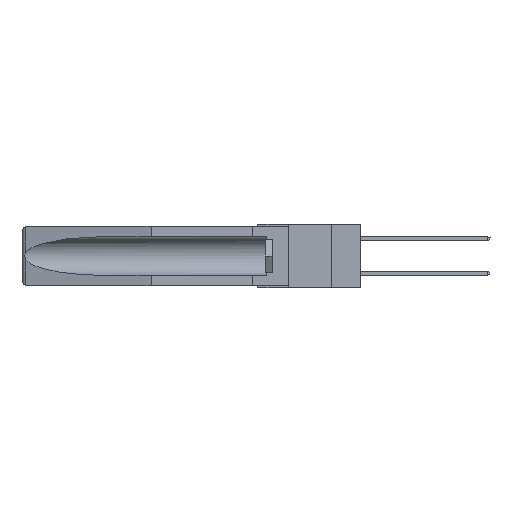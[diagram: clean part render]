
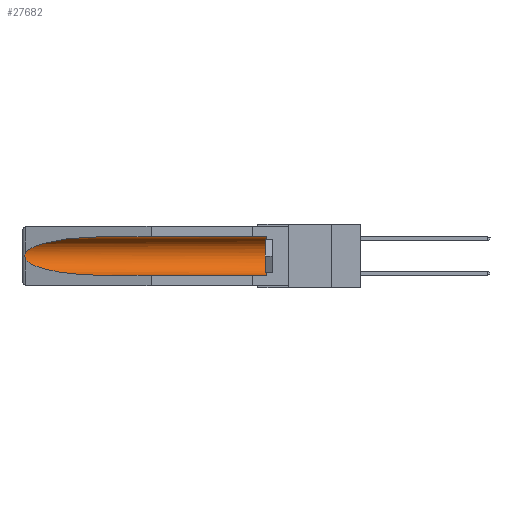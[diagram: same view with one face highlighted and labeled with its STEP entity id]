
A CAD part, left-side view. The second image highlights one B-rep face of the part: STEP entity #27682.
In plain terms, the highlighted cylindrical face has radius 2.857 mm (diameter 5.715 mm), a partial arc.
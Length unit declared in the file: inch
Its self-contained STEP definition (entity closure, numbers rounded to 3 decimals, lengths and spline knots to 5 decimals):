
#63 = DIRECTION ( 'NONE',  ( 0., 1., 0. ) ) ;
#552 = CARTESIAN_POINT ( 'NONE',  ( 0.26537, 1.52718, -0.14972 ) ) ;
#564 = VERTEX_POINT ( 'NONE', #11692 ) ;
#1030 = CARTESIAN_POINT ( 'NONE',  ( 0.155, 0.126, -0.1715 ) ) ;
#1055 = ORIENTED_EDGE ( 'NONE', *, *, #6810, .T. ) ;
#1767 = VECTOR ( 'NONE', #63, 39.37008 ) ;
#1790 = ORIENTED_EDGE ( 'NONE', *, *, #19534, .T. ) ;
#1991 = LINE ( 'NONE', #5428, #10099 ) ;
#2625 = EDGE_LOOP ( 'NONE', ( #1055, #1790, #20325, #8831, #15726, #8059 ) ) ;
#3124 = CARTESIAN_POINT ( 'NONE',  ( 0.26597, 1.5296, -0.19026 ) ) ;
#3127 = FACE_OUTER_BOUND ( 'NONE', #2625, .T. ) ;
#4178 = CARTESIAN_POINT ( 'NONE',  ( 0.155, 0.126, -0.059 ) ) ;
#4652 = CARTESIAN_POINT ( 'NONE',  ( 0.21114, 1.30732, -0.059 ) ) ;
#4722 = B_SPLINE_CURVE_WITH_KNOTS ( 'NONE', 3,
 ( #552, #7975, #10685, #25321, #10466, #5264, #12987, #22663, #3124, #30252 ),
 .UNSPECIFIED., .F., .F.,
 ( 4, 2, 2, 2, 4 ),
 ( 0., 0.00029, 0.00058, 0.00087, 0.00117 ),
 .UNSPECIFIED. ) ;
#5264 = CARTESIAN_POINT ( 'NONE',  ( 0.2675, 1.53308, -0.17534 ) ) ;
#5428 = CARTESIAN_POINT ( 'NONE',  ( 0.155, -0.30754, -0.284 ) ) ;
#5488 = EDGE_CURVE ( 'NONE', #23684, #7518, #30255, .T. ) ;
#5965 = DIRECTION ( 'NONE',  ( 0., 0., 1. ) ) ;
#6353 = VERTEX_POINT ( 'NONE', #21353 ) ;
#6810 = EDGE_CURVE ( 'NONE', #564, #6353, #24814, .T. ) ;
#7254 = CARTESIAN_POINT ( 'NONE',  ( 0.155, 0.126, -0.284 ) ) ;
#7518 = VERTEX_POINT ( 'NONE', #4178 ) ;
#7650 = AXIS2_PLACEMENT_3D ( 'NONE', #16590, #11822, #24084 ) ;
#7975 = CARTESIAN_POINT ( 'NONE',  ( 0.26597, 1.52961, -0.15275 ) ) ;
#8059 = ORIENTED_EDGE ( 'NONE', *, *, #25004, .T. ) ;
#8831 = ORIENTED_EDGE ( 'NONE', *, *, #16434, .F. ) ;
#9726 = CARTESIAN_POINT ( 'NONE',  ( 0.155, 1.07973, -0.059 ) ) ;
#10099 = VECTOR ( 'NONE', #10294, 39.37008 ) ;
#10294 = DIRECTION ( 'NONE',  ( 0., 1., 0. ) ) ;
#10466 = CARTESIAN_POINT ( 'NONE',  ( 0.2675, 1.53308, -0.16763 ) ) ;
#10685 = CARTESIAN_POINT ( 'NONE',  ( 0.26654, 1.53092, -0.15636 ) ) ;
#11692 = CARTESIAN_POINT ( 'NONE',  ( 0.155, 1.07973, -0.059 ) ) ;
#11822 = DIRECTION ( 'NONE',  ( 0., 1., 0. ) ) ;
#12987 = CARTESIAN_POINT ( 'NONE',  ( 0.2673, 1.53269, -0.17917 ) ) ;
#13715 = CARTESIAN_POINT ( 'NONE',  ( 0.21114, 1.30732, -0.284 ) ) ;
#13816 = CARTESIAN_POINT ( 'NONE',  ( 0.155, 1.07973, -0.284 ) ) ;
#14233 = VERTEX_POINT ( 'NONE', #27488 ) ;
#15195 = CARTESIAN_POINT ( 'NONE',  ( 0.155, -0.30754, -0.059 ) ) ;
#15726 = ORIENTED_EDGE ( 'NONE', *, *, #5488, .T. ) ;
#16235 = CARTESIAN_POINT ( 'NONE',  ( 0.155, 1.07973, -0.284 ) ) ;
#16434 = EDGE_CURVE ( 'NONE', #23684, #21616, #1991, .T. ) ;
#16590 = CARTESIAN_POINT ( 'NONE',  ( 0.155, -0.30754, -0.1715 ) ) ;
#16810 = CARTESIAN_POINT ( 'NONE',  ( 0.26537, 1.52718, -0.14972 ) ) ;
#17638 = LINE ( 'NONE', #15195, #1767 ) ;
#18564 = DIRECTION ( 'NONE',  ( 0., -1., 0. ) ) ;
#19534 = EDGE_CURVE ( 'NONE', #6353, #14233, #4722, .T. ) ;
#19648 =( BOUNDED_CURVE ( )  B_SPLINE_CURVE ( 3, ( #20902, #28586, #13715, #13816 ),
 .UNSPECIFIED., .F., .F. ) 
 B_SPLINE_CURVE_WITH_KNOTS ( ( 4, 4 ),
 ( 0.1948, 1.5708 ),
 .UNSPECIFIED. ) 
 CURVE ( )  GEOMETRIC_REPRESENTATION_ITEM ( )  RATIONAL_B_SPLINE_CURVE ( ( 1., 0.848, 0.848, 1. ) ) 
 REPRESENTATION_ITEM ( '' )  );
#20325 = ORIENTED_EDGE ( 'NONE', *, *, #24693, .T. ) ;
#20902 = CARTESIAN_POINT ( 'NONE',  ( 0.26537, 1.52718, -0.19328 ) ) ;
#21353 = CARTESIAN_POINT ( 'NONE',  ( 0.26537, 1.52718, -0.14972 ) ) ;
#21616 = VERTEX_POINT ( 'NONE', #16235 ) ;
#22663 = CARTESIAN_POINT ( 'NONE',  ( 0.26655, 1.53094, -0.18657 ) ) ;
#23684 = VERTEX_POINT ( 'NONE', #7254 ) ;
#23705 = CYLINDRICAL_SURFACE ( 'NONE', #7650, 0.1125 ) ;
#24084 = DIRECTION ( 'NONE',  ( 0., 0., 1. ) ) ;
#24693 = EDGE_CURVE ( 'NONE', #14233, #21616, #19648, .T. ) ;
#24814 =( BOUNDED_CURVE ( )  B_SPLINE_CURVE ( 3, ( #9726, #4652, #29293, #16810 ),
 .UNSPECIFIED., .F., .F. ) 
 B_SPLINE_CURVE_WITH_KNOTS ( ( 4, 4 ),
 ( 4.71239, 6.08839 ),
 .UNSPECIFIED. ) 
 CURVE ( )  GEOMETRIC_REPRESENTATION_ITEM ( )  RATIONAL_B_SPLINE_CURVE ( ( 1., 0.848, 0.848, 1. ) ) 
 REPRESENTATION_ITEM ( '' )  );
#25004 = EDGE_CURVE ( 'NONE', #7518, #564, #17638, .T. ) ;
#25321 = CARTESIAN_POINT ( 'NONE',  ( 0.2673, 1.5327, -0.16383 ) ) ;
#26771 = AXIS2_PLACEMENT_3D ( 'NONE', #1030, #18564, #5965 ) ;
#27488 = CARTESIAN_POINT ( 'NONE',  ( 0.26537, 1.52718, -0.19328 ) ) ;
#27682 = ADVANCED_FACE ( 'NONE', ( #3127 ), #23705, .F. ) ;
#28586 = CARTESIAN_POINT ( 'NONE',  ( 0.25451, 1.48313, -0.24835 ) ) ;
#29293 = CARTESIAN_POINT ( 'NONE',  ( 0.25451, 1.48313, -0.09465 ) ) ;
#30252 = CARTESIAN_POINT ( 'NONE',  ( 0.26537, 1.52718, -0.19328 ) ) ;
#30255 = CIRCLE ( 'NONE', #26771, 0.1125 ) ;
